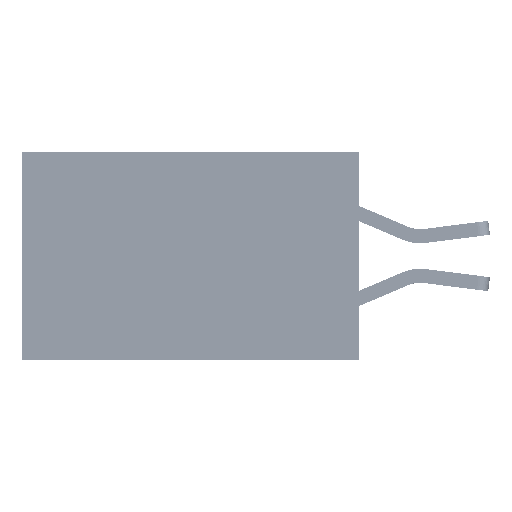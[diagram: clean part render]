
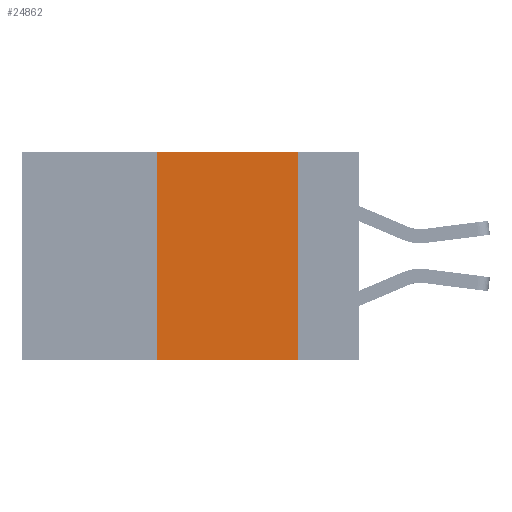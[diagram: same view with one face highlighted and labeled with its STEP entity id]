
A CAD part, left-side view. The second image highlights one B-rep face of the part: STEP entity #24862.
In plain terms, the highlighted planar face has unit normal (-1, 0, 0).
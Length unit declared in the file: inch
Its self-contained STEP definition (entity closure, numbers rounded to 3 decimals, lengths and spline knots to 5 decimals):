
#3013 = EDGE_CURVE ( 'NONE', #24367, #31666, #24461, .T. ) ;
#3349 = VERTEX_POINT ( 'NONE', #24816 ) ;
#4555 = ORIENTED_EDGE ( 'NONE', *, *, #3013, .F. ) ;
#5107 = DIRECTION ( 'NONE',  ( 1., 0., 0. ) ) ;
#9087 = LINE ( 'NONE', #17667, #13302 ) ;
#9215 = DIRECTION ( 'NONE',  ( 0., 0., -1. ) ) ;
#10991 = VECTOR ( 'NONE', #32517, 39.37008 ) ;
#11434 = EDGE_CURVE ( 'NONE', #31666, #15369, #9087, .T. ) ;
#13302 = VECTOR ( 'NONE', #9215, 39.37008 ) ;
#14612 = CARTESIAN_POINT ( 'NONE',  ( 0., 0.6, 0. ) ) ;
#15369 = VERTEX_POINT ( 'NONE', #35437 ) ;
#15573 = LINE ( 'NONE', #31648, #35536 ) ;
#16916 = DIRECTION ( 'NONE',  ( 0., 0., 1. ) ) ;
#16941 = CARTESIAN_POINT ( 'NONE',  ( 0., 0.6, 0. ) ) ;
#17033 = VECTOR ( 'NONE', #16916, 39.37008 ) ;
#17478 = EDGE_CURVE ( 'NONE', #3349, #15369, #15573, .T. ) ;
#17667 = CARTESIAN_POINT ( 'NONE',  ( 0., 0.11, 0. ) ) ;
#19850 = CARTESIAN_POINT ( 'NONE',  ( 0., 0.11, 0. ) ) ;
#20713 = CARTESIAN_POINT ( 'NONE',  ( 0., 0.36, 0. ) ) ;
#21547 = ORIENTED_EDGE ( 'NONE', *, *, #17478, .T. ) ;
#24367 = VERTEX_POINT ( 'NONE', #20713 ) ;
#24461 = LINE ( 'NONE', #14612, #10991 ) ;
#24816 = CARTESIAN_POINT ( 'NONE',  ( 0., 0.36, -0.37 ) ) ;
#24862 = ADVANCED_FACE ( 'NONE', ( #37457 ), #34480, .F. ) ;
#25787 = DIRECTION ( 'NONE',  ( 0., -1., 0. ) ) ;
#26585 = ORIENTED_EDGE ( 'NONE', *, *, #11434, .F. ) ;
#31648 = CARTESIAN_POINT ( 'NONE',  ( 0., 0.6, -0.37 ) ) ;
#31666 = VERTEX_POINT ( 'NONE', #19850 ) ;
#32232 = AXIS2_PLACEMENT_3D ( 'NONE', #16941, #5107, #37591 ) ;
#32517 = DIRECTION ( 'NONE',  ( 0., -1., 0. ) ) ;
#33889 = ORIENTED_EDGE ( 'NONE', *, *, #35284, .F. ) ;
#34480 = PLANE ( 'NONE',  #32232 ) ;
#35284 = EDGE_CURVE ( 'NONE', #3349, #24367, #37003, .T. ) ;
#35437 = CARTESIAN_POINT ( 'NONE',  ( 0., 0.11, -0.37 ) ) ;
#35536 = VECTOR ( 'NONE', #25787, 39.37008 ) ;
#35949 = EDGE_LOOP ( 'NONE', ( #26585, #4555, #33889, #21547 ) ) ;
#37003 = LINE ( 'NONE', #37561, #17033 ) ;
#37457 = FACE_OUTER_BOUND ( 'NONE', #35949, .T. ) ;
#37561 = CARTESIAN_POINT ( 'NONE',  ( 0., 0.36, 0. ) ) ;
#37591 = DIRECTION ( 'NONE',  ( 0., 0., -1. ) ) ;
